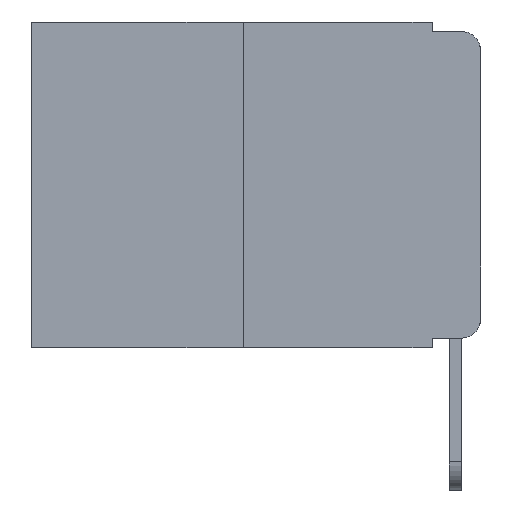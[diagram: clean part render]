
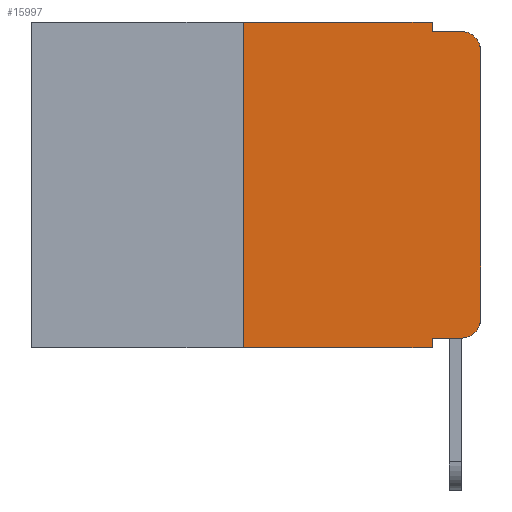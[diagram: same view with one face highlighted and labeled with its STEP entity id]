
A CAD part, left-side view. The second image highlights one B-rep face of the part: STEP entity #15997.
In plain terms, the highlighted planar face has unit normal (-1, 0, 0).
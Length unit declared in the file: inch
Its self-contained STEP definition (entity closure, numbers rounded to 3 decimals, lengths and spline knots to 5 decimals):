
#25 = EDGE_CURVE ( 'NONE', #16823, #13169, #15633, .T. ) ;
#159 = DIRECTION ( 'NONE',  ( 0., -1., 0. ) ) ;
#172 = ORIENTED_EDGE ( 'NONE', *, *, #5729, .T. ) ;
#218 = ORIENTED_EDGE ( 'NONE', *, *, #6819, .F. ) ;
#461 = ORIENTED_EDGE ( 'NONE', *, *, #7902, .F. ) ;
#553 = LINE ( 'NONE', #11144, #15995 ) ;
#571 = CARTESIAN_POINT ( 'NONE',  ( 0., 0.02, -0.01 ) ) ;
#1182 = ORIENTED_EDGE ( 'NONE', *, *, #18906, .F. ) ;
#1434 = ORIENTED_EDGE ( 'NONE', *, *, #8852, .F. ) ;
#1727 = CARTESIAN_POINT ( 'NONE',  ( 0., 0.473, -0.343 ) ) ;
#1756 = DIRECTION ( 'NONE',  ( 0., 0., -1. ) ) ;
#2338 = CIRCLE ( 'NONE', #3175, 0.02 ) ;
#2778 = ORIENTED_EDGE ( 'NONE', *, *, #14308, .T. ) ;
#2811 = CARTESIAN_POINT ( 'NONE',  ( 0., 0., -0.313 ) ) ;
#3175 = AXIS2_PLACEMENT_3D ( 'NONE', #16827, #8686, #18201 ) ;
#3363 = EDGE_LOOP ( 'NONE', ( #7475, #172, #218, #461, #1182, #1434, #5177, #8040, #10196, #2778 ) ) ;
#3443 = CARTESIAN_POINT ( 'NONE',  ( 0., 0.473, 0. ) ) ;
#3546 = EDGE_CURVE ( 'NONE', #5924, #9474, #17949, .T. ) ;
#3771 = VECTOR ( 'NONE', #18446, 39.37008 ) ;
#4423 = CARTESIAN_POINT ( 'NONE',  ( 0., 0.051, -0.01 ) ) ;
#4545 = VERTEX_POINT ( 'NONE', #571 ) ;
#4638 = CARTESIAN_POINT ( 'NONE',  ( 0., 0., 0. ) ) ;
#5177 = ORIENTED_EDGE ( 'NONE', *, *, #25, .T. ) ;
#5339 = DIRECTION ( 'NONE',  ( 0., 0., -1. ) ) ;
#5729 = EDGE_CURVE ( 'NONE', #9474, #4545, #2338, .T. ) ;
#5924 = VERTEX_POINT ( 'NONE', #2811 ) ;
#5950 = CARTESIAN_POINT ( 'NONE',  ( 0., 0.02, -0.313 ) ) ;
#6041 = DIRECTION ( 'NONE',  ( 0., -1., 0. ) ) ;
#6484 = DIRECTION ( 'NONE',  ( 0., -1., 0. ) ) ;
#6696 = DIRECTION ( 'NONE',  ( 0., -1., 0. ) ) ;
#6796 = DIRECTION ( 'NONE',  ( 0., 0., -1. ) ) ;
#6819 = EDGE_CURVE ( 'NONE', #16547, #4545, #6970, .T. ) ;
#6970 = LINE ( 'NONE', #4423, #10328 ) ;
#6994 = VECTOR ( 'NONE', #1756, 39.37008 ) ;
#7475 = ORIENTED_EDGE ( 'NONE', *, *, #3546, .T. ) ;
#7565 = DIRECTION ( 'NONE',  ( 0., 0., -1. ) ) ;
#7902 = EDGE_CURVE ( 'NONE', #11877, #16547, #553, .T. ) ;
#8040 = ORIENTED_EDGE ( 'NONE', *, *, #11562, .F. ) ;
#8425 = CARTESIAN_POINT ( 'NONE',  ( 0., 0.473, 0. ) ) ;
#8686 = DIRECTION ( 'NONE',  ( -1., 0., 0. ) ) ;
#8852 = EDGE_CURVE ( 'NONE', #16823, #9152, #11689, .T. ) ;
#8927 = VERTEX_POINT ( 'NONE', #10438 ) ;
#9152 = VERTEX_POINT ( 'NONE', #18900 ) ;
#9474 = VERTEX_POINT ( 'NONE', #9952 ) ;
#9699 = CARTESIAN_POINT ( 'NONE',  ( 0., 0.051, 0. ) ) ;
#9920 = LINE ( 'NONE', #8425, #16720 ) ;
#9952 = CARTESIAN_POINT ( 'NONE',  ( 0., 0., -0.03 ) ) ;
#10196 = ORIENTED_EDGE ( 'NONE', *, *, #12497, .T. ) ;
#10328 = VECTOR ( 'NONE', #6041, 39.37008 ) ;
#10438 = CARTESIAN_POINT ( 'NONE',  ( 0., 0.051, -0.333 ) ) ;
#10931 = LINE ( 'NONE', #14847, #14568 ) ;
#11144 = CARTESIAN_POINT ( 'NONE',  ( 0., 0.051, 0. ) ) ;
#11562 = EDGE_CURVE ( 'NONE', #8927, #13169, #14821, .T. ) ;
#11689 = LINE ( 'NONE', #17110, #3771 ) ;
#11877 = VERTEX_POINT ( 'NONE', #17194 ) ;
#12205 = AXIS2_PLACEMENT_3D ( 'NONE', #3443, #15114, #6796 ) ;
#12497 = EDGE_CURVE ( 'NONE', #8927, #17006, #10931, .T. ) ;
#13169 = VERTEX_POINT ( 'NONE', #16322 ) ;
#13770 = PLANE ( 'NONE',  #12205 ) ;
#13911 = VECTOR ( 'NONE', #16010, 39.37008 ) ;
#14308 = EDGE_CURVE ( 'NONE', #17006, #5924, #14536, .T. ) ;
#14536 = CIRCLE ( 'NONE', #19065, 0.02 ) ;
#14568 = VECTOR ( 'NONE', #6484, 39.37008 ) ;
#14682 = FACE_OUTER_BOUND ( 'NONE', #3363, .T. ) ;
#14749 = CARTESIAN_POINT ( 'NONE',  ( 0., 0.02, -0.333 ) ) ;
#14765 = CARTESIAN_POINT ( 'NONE',  ( 0., 0.051, -0.01 ) ) ;
#14821 = LINE ( 'NONE', #9699, #6994 ) ;
#14847 = CARTESIAN_POINT ( 'NONE',  ( 0., 0.051, -0.333 ) ) ;
#15114 = DIRECTION ( 'NONE',  ( 1., 0., 0. ) ) ;
#15633 = LINE ( 'NONE', #1727, #16079 ) ;
#15777 = DIRECTION ( 'NONE',  ( -1., 0., 0. ) ) ;
#15995 = VECTOR ( 'NONE', #5339, 39.37008 ) ;
#15997 = ADVANCED_FACE ( 'NONE', ( #14682 ), #13770, .F. ) ;
#16010 = DIRECTION ( 'NONE',  ( 0., 0., 1. ) ) ;
#16079 = VECTOR ( 'NONE', #6696, 39.37008 ) ;
#16322 = CARTESIAN_POINT ( 'NONE',  ( 0., 0.051, -0.343 ) ) ;
#16547 = VERTEX_POINT ( 'NONE', #14765 ) ;
#16720 = VECTOR ( 'NONE', #159, 39.37008 ) ;
#16823 = VERTEX_POINT ( 'NONE', #18198 ) ;
#16827 = CARTESIAN_POINT ( 'NONE',  ( 0., 0.02, -0.03 ) ) ;
#17006 = VERTEX_POINT ( 'NONE', #14749 ) ;
#17110 = CARTESIAN_POINT ( 'NONE',  ( 0., 0.25, 0. ) ) ;
#17194 = CARTESIAN_POINT ( 'NONE',  ( 0., 0.051, 0. ) ) ;
#17949 = LINE ( 'NONE', #4638, #13911 ) ;
#18198 = CARTESIAN_POINT ( 'NONE',  ( 0., 0.25, -0.343 ) ) ;
#18201 = DIRECTION ( 'NONE',  ( 0., 0., -1. ) ) ;
#18446 = DIRECTION ( 'NONE',  ( 0., 0., 1. ) ) ;
#18900 = CARTESIAN_POINT ( 'NONE',  ( 0., 0.25, 0. ) ) ;
#18906 = EDGE_CURVE ( 'NONE', #9152, #11877, #9920, .T. ) ;
#19065 = AXIS2_PLACEMENT_3D ( 'NONE', #5950, #15777, #7565 ) ;
